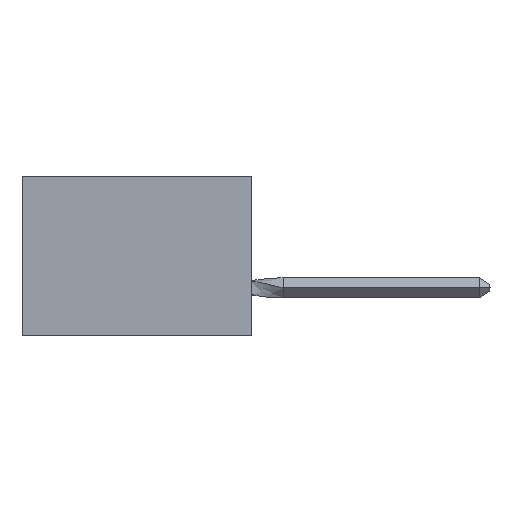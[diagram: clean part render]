
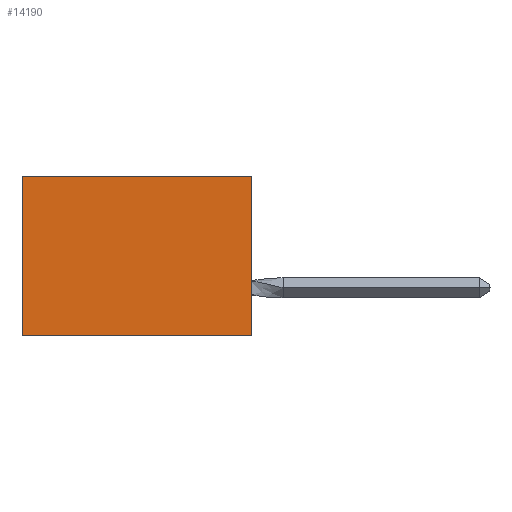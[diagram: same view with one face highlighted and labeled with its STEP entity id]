
A CAD part, left-side view. The second image highlights one B-rep face of the part: STEP entity #14190.
In plain terms, the highlighted planar face has unit normal (-1, 0, 0).
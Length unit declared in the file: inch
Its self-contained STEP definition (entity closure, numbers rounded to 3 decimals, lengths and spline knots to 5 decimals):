
#635 = LINE ( 'NONE', #16474, #9458 ) ;
#2339 = VERTEX_POINT ( 'NONE', #3553 ) ;
#3553 = CARTESIAN_POINT ( 'NONE',  ( 0.305, 0., -0.5 ) ) ;
#3674 = CARTESIAN_POINT ( 'NONE',  ( 0.305, 0., -0.5 ) ) ;
#5147 = CARTESIAN_POINT ( 'NONE',  ( 0.305, 0., 0. ) ) ;
#6601 = CARTESIAN_POINT ( 'NONE',  ( 0.305, 0., -0.5 ) ) ;
#6757 = EDGE_LOOP ( 'NONE', ( #19627, #16244, #18671, #21060 ) ) ;
#6773 = DIRECTION ( 'NONE',  ( 0., 1., 0. ) ) ;
#7289 = VECTOR ( 'NONE', #6773, 39.37008 ) ;
#7387 = EDGE_CURVE ( 'NONE', #17521, #13960, #635, .T. ) ;
#8230 = EDGE_CURVE ( 'NONE', #17521, #2339, #20501, .T. ) ;
#9458 = VECTOR ( 'NONE', #14745, 39.37008 ) ;
#9529 = VERTEX_POINT ( 'NONE', #10644 ) ;
#10614 = CARTESIAN_POINT ( 'NONE',  ( 0.305, 0.72, -0.5 ) ) ;
#10644 = CARTESIAN_POINT ( 'NONE',  ( 0.305, 0.72, -0.5 ) ) ;
#10784 = DIRECTION ( 'NONE',  ( 1., 0., 0. ) ) ;
#11227 = EDGE_CURVE ( 'NONE', #13960, #9529, #22333, .T. ) ;
#12135 = LINE ( 'NONE', #6601, #7289 ) ;
#12315 = DIRECTION ( 'NONE',  ( 0., 0., -1. ) ) ;
#13960 = VERTEX_POINT ( 'NONE', #17004 ) ;
#14095 = EDGE_CURVE ( 'NONE', #2339, #9529, #12135, .T. ) ;
#14190 = ADVANCED_FACE ( 'NONE', ( #20657 ), #21455, .F. ) ;
#14460 = AXIS2_PLACEMENT_3D ( 'NONE', #21373, #10784, #12315 ) ;
#14632 = VECTOR ( 'NONE', #23261, 39.37008 ) ;
#14698 = DIRECTION ( 'NONE',  ( 0., 0., -1. ) ) ;
#14745 = DIRECTION ( 'NONE',  ( 0., 1., 0. ) ) ;
#15947 = VECTOR ( 'NONE', #14698, 39.37008 ) ;
#16244 = ORIENTED_EDGE ( 'NONE', *, *, #14095, .F. ) ;
#16474 = CARTESIAN_POINT ( 'NONE',  ( 0.305, 0., 0. ) ) ;
#17004 = CARTESIAN_POINT ( 'NONE',  ( 0.305, 0.72, 0. ) ) ;
#17521 = VERTEX_POINT ( 'NONE', #5147 ) ;
#18671 = ORIENTED_EDGE ( 'NONE', *, *, #8230, .F. ) ;
#19627 = ORIENTED_EDGE ( 'NONE', *, *, #11227, .T. ) ;
#20501 = LINE ( 'NONE', #3674, #15947 ) ;
#20657 = FACE_OUTER_BOUND ( 'NONE', #6757, .T. ) ;
#21060 = ORIENTED_EDGE ( 'NONE', *, *, #7387, .T. ) ;
#21373 = CARTESIAN_POINT ( 'NONE',  ( 0.305, 0., -0.5 ) ) ;
#21455 = PLANE ( 'NONE',  #14460 ) ;
#22333 = LINE ( 'NONE', #10614, #14632 ) ;
#23261 = DIRECTION ( 'NONE',  ( 0., 0., -1. ) ) ;
